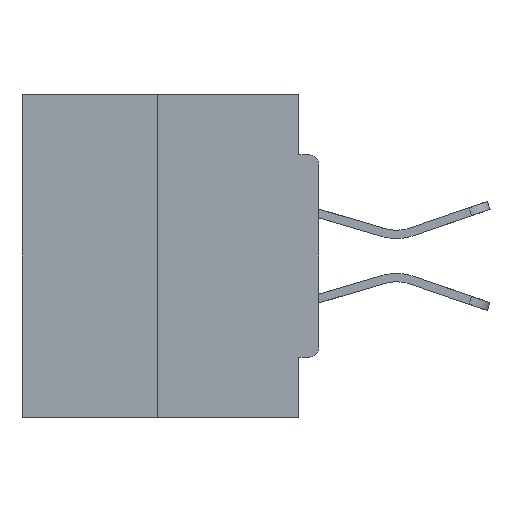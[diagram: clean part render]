
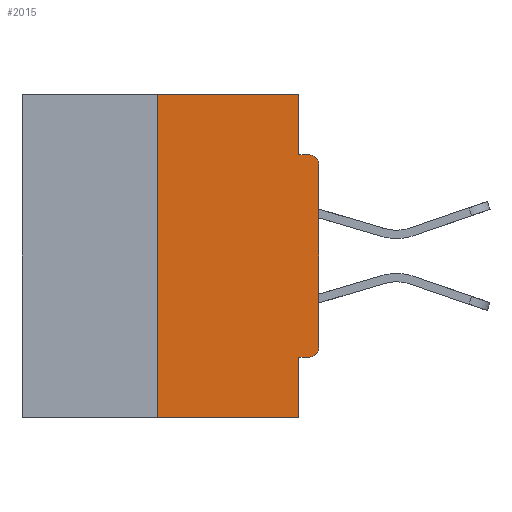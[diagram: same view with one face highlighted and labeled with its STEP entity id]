
A CAD part, left-side view. The second image highlights one B-rep face of the part: STEP entity #2015.
In plain terms, the highlighted planar face has unit normal (-1, 0, 0).
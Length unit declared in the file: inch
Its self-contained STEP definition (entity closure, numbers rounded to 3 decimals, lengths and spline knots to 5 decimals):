
#289 = EDGE_CURVE ( 'NONE', #29199, #24686, #22436, .T. ) ;
#334 = EDGE_CURVE ( 'NONE', #24686, #25262, #4704, .T. ) ;
#1763 = CARTESIAN_POINT ( 'NONE',  ( 0., 0.46, 0. ) ) ;
#2015 = ADVANCED_FACE ( 'NONE', ( #10295 ), #19377, .F. ) ;
#2090 = CARTESIAN_POINT ( 'NONE',  ( 0., 0.015, -0.3915 ) ) ;
#2253 = VECTOR ( 'NONE', #13956, 39.37008 ) ;
#2672 = CARTESIAN_POINT ( 'NONE',  ( 0., 0., -0.4065 ) ) ;
#3387 = CIRCLE ( 'NONE', #28000, 0.015 ) ;
#4081 = CARTESIAN_POINT ( 'NONE',  ( 0., 0.031, 0. ) ) ;
#4704 = LINE ( 'NONE', #28650, #22855 ) ;
#5390 = ORIENTED_EDGE ( 'NONE', *, *, #14894, .T. ) ;
#5533 = CARTESIAN_POINT ( 'NONE',  ( 0., 0.031, 0. ) ) ;
#6097 = CARTESIAN_POINT ( 'NONE',  ( 0., 0.031, -0.4065 ) ) ;
#6130 = CIRCLE ( 'NONE', #25676, 0.015 ) ;
#6240 = CARTESIAN_POINT ( 'NONE',  ( 0., 0., 0. ) ) ;
#6930 = VERTEX_POINT ( 'NONE', #32060 ) ;
#7336 = CARTESIAN_POINT ( 'NONE',  ( 0., 0.031, -0.0935 ) ) ;
#8306 = CARTESIAN_POINT ( 'NONE',  ( 0., 0., -0.1085 ) ) ;
#8467 = CARTESIAN_POINT ( 'NONE',  ( 0., 0.46, 0. ) ) ;
#9315 = VERTEX_POINT ( 'NONE', #18730 ) ;
#9780 = EDGE_CURVE ( 'NONE', #9315, #19421, #28851, .T. ) ;
#10295 = FACE_OUTER_BOUND ( 'NONE', #20882, .T. ) ;
#10332 = VECTOR ( 'NONE', #11027, 39.37008 ) ;
#10581 = VECTOR ( 'NONE', #29026, 39.37008 ) ;
#10740 = DIRECTION ( 'NONE',  ( 0., -1., 0. ) ) ;
#11027 = DIRECTION ( 'NONE',  ( 0., -1., 0. ) ) ;
#11621 = CARTESIAN_POINT ( 'NONE',  ( 0., 0., -0.3915 ) ) ;
#12230 = CARTESIAN_POINT ( 'NONE',  ( 0., 0.015, -0.1085 ) ) ;
#12683 = EDGE_CURVE ( 'NONE', #19384, #19421, #14872, .T. ) ;
#12855 = VECTOR ( 'NONE', #20259, 39.37008 ) ;
#12873 = ORIENTED_EDGE ( 'NONE', *, *, #12683, .F. ) ;
#12988 = DIRECTION ( 'NONE',  ( 0., 0., -1. ) ) ;
#13161 = AXIS2_PLACEMENT_3D ( 'NONE', #1763, #29507, #32154 ) ;
#13321 = ORIENTED_EDGE ( 'NONE', *, *, #289, .F. ) ;
#13670 = ORIENTED_EDGE ( 'NONE', *, *, #28846, .F. ) ;
#13764 = CARTESIAN_POINT ( 'NONE',  ( 0., 0.46, -0.5 ) ) ;
#13787 = CARTESIAN_POINT ( 'NONE',  ( 0., 0.015, -0.4065 ) ) ;
#13956 = DIRECTION ( 'NONE',  ( 0., 0., -1. ) ) ;
#14157 = CARTESIAN_POINT ( 'NONE',  ( 0., 0.031, -0.5 ) ) ;
#14872 = LINE ( 'NONE', #28692, #2253 ) ;
#14894 = EDGE_CURVE ( 'NONE', #20076, #16634, #3387, .T. ) ;
#15489 = EDGE_CURVE ( 'NONE', #32093, #25262, #6130, .T. ) ;
#15820 = ORIENTED_EDGE ( 'NONE', *, *, #334, .F. ) ;
#16634 = VERTEX_POINT ( 'NONE', #11621 ) ;
#18702 = ORIENTED_EDGE ( 'NONE', *, *, #9780, .T. ) ;
#18703 = DIRECTION ( 'NONE',  ( 0., -1., 0. ) ) ;
#18730 = CARTESIAN_POINT ( 'NONE',  ( 0., 0.25, -0.5 ) ) ;
#18976 = LINE ( 'NONE', #8467, #24107 ) ;
#19377 = PLANE ( 'NONE',  #13161 ) ;
#19384 = VERTEX_POINT ( 'NONE', #6097 ) ;
#19421 = VERTEX_POINT ( 'NONE', #14157 ) ;
#20076 = VERTEX_POINT ( 'NONE', #13787 ) ;
#20259 = DIRECTION ( 'NONE',  ( 0., 1., 0. ) ) ;
#20882 = EDGE_LOOP ( 'NONE', ( #21472, #27252, #18702, #12873, #13670, #5390, #25069, #26587, #15820, #13321 ) ) ;
#21406 = EDGE_CURVE ( 'NONE', #9315, #6930, #28419, .T. ) ;
#21453 = EDGE_CURVE ( 'NONE', #6930, #29199, #18976, .T. ) ;
#21472 = ORIENTED_EDGE ( 'NONE', *, *, #21453, .F. ) ;
#21940 = CARTESIAN_POINT ( 'NONE',  ( 0., 0.015, -0.0935 ) ) ;
#22249 = DIRECTION ( 'NONE',  ( 0., 0., -1. ) ) ;
#22436 = LINE ( 'NONE', #5533, #26374 ) ;
#22855 = VECTOR ( 'NONE', #10740, 39.37008 ) ;
#24107 = VECTOR ( 'NONE', #18703, 39.37008 ) ;
#24686 = VERTEX_POINT ( 'NONE', #7336 ) ;
#25068 = LINE ( 'NONE', #2672, #12855 ) ;
#25069 = ORIENTED_EDGE ( 'NONE', *, *, #27847, .T. ) ;
#25262 = VERTEX_POINT ( 'NONE', #21940 ) ;
#25676 = AXIS2_PLACEMENT_3D ( 'NONE', #12230, #32347, #12988 ) ;
#26374 = VECTOR ( 'NONE', #31076, 39.37008 ) ;
#26398 = CARTESIAN_POINT ( 'NONE',  ( 0., 0.25, 0. ) ) ;
#26587 = ORIENTED_EDGE ( 'NONE', *, *, #15489, .T. ) ;
#26680 = LINE ( 'NONE', #6240, #10581 ) ;
#27252 = ORIENTED_EDGE ( 'NONE', *, *, #21406, .F. ) ;
#27847 = EDGE_CURVE ( 'NONE', #16634, #32093, #26680, .T. ) ;
#28000 = AXIS2_PLACEMENT_3D ( 'NONE', #2090, #30058, #22249 ) ;
#28045 = VECTOR ( 'NONE', #28829, 39.37008 ) ;
#28419 = LINE ( 'NONE', #26398, #28045 ) ;
#28650 = CARTESIAN_POINT ( 'NONE',  ( 0., 0., -0.0935 ) ) ;
#28692 = CARTESIAN_POINT ( 'NONE',  ( 0., 0.031, -0.5 ) ) ;
#28829 = DIRECTION ( 'NONE',  ( 0., 0., 1. ) ) ;
#28846 = EDGE_CURVE ( 'NONE', #20076, #19384, #25068, .T. ) ;
#28851 = LINE ( 'NONE', #13764, #10332 ) ;
#29026 = DIRECTION ( 'NONE',  ( 0., 0., 1. ) ) ;
#29199 = VERTEX_POINT ( 'NONE', #4081 ) ;
#29507 = DIRECTION ( 'NONE',  ( 1., 0., 0. ) ) ;
#30058 = DIRECTION ( 'NONE',  ( -1., 0., 0. ) ) ;
#31076 = DIRECTION ( 'NONE',  ( 0., 0., -1. ) ) ;
#32060 = CARTESIAN_POINT ( 'NONE',  ( 0., 0.25, 0. ) ) ;
#32093 = VERTEX_POINT ( 'NONE', #8306 ) ;
#32154 = DIRECTION ( 'NONE',  ( 0., 0., -1. ) ) ;
#32347 = DIRECTION ( 'NONE',  ( -1., 0., 0. ) ) ;
